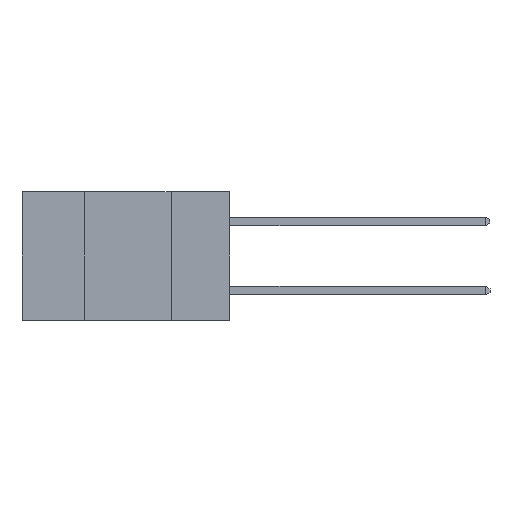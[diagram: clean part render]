
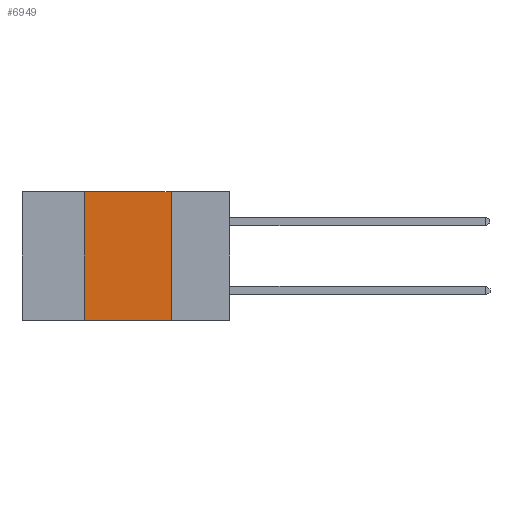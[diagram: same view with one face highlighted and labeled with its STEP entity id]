
A CAD part, left-side view. The second image highlights one B-rep face of the part: STEP entity #6949.
In plain terms, the highlighted planar face has unit normal (-1, 0, 0).
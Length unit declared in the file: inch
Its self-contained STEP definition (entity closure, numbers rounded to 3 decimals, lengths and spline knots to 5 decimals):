
#472 = VECTOR ( 'NONE', #587, 39.37008 ) ;
#587 = DIRECTION ( 'NONE',  ( 0., 0., -1. ) ) ;
#856 = CARTESIAN_POINT ( 'NONE',  ( 0., 0.6, 0. ) ) ;
#1259 = ORIENTED_EDGE ( 'NONE', *, *, #6615, .F. ) ;
#1535 = CARTESIAN_POINT ( 'NONE',  ( 0., 0.42, -0.37 ) ) ;
#1783 = VECTOR ( 'NONE', #5575, 39.37008 ) ;
#3051 = CARTESIAN_POINT ( 'NONE',  ( 0., 0.42, -0.37 ) ) ;
#3901 = DIRECTION ( 'NONE',  ( 0., -1., 0. ) ) ;
#3947 = LINE ( 'NONE', #3051, #8291 ) ;
#4255 = ORIENTED_EDGE ( 'NONE', *, *, #5945, .F. ) ;
#4301 = DIRECTION ( 'NONE',  ( 1., 0., 0. ) ) ;
#4339 = VERTEX_POINT ( 'NONE', #1535 ) ;
#4777 = LINE ( 'NONE', #9159, #472 ) ;
#5204 = EDGE_CURVE ( 'NONE', #4339, #5522, #6720, .T. ) ;
#5350 = EDGE_CURVE ( 'NONE', #5360, #5522, #4777, .T. ) ;
#5360 = VERTEX_POINT ( 'NONE', #7502 ) ;
#5522 = VERTEX_POINT ( 'NONE', #11032 ) ;
#5575 = DIRECTION ( 'NONE',  ( 0., -1., 0. ) ) ;
#5828 = ORIENTED_EDGE ( 'NONE', *, *, #5204, .T. ) ;
#5945 = EDGE_CURVE ( 'NONE', #4339, #7192, #3947, .T. ) ;
#6615 = EDGE_CURVE ( 'NONE', #7192, #5360, #10874, .T. ) ;
#6720 = LINE ( 'NONE', #9827, #1783 ) ;
#6949 = ADVANCED_FACE ( 'NONE', ( #9704 ), #9466, .F. ) ;
#7192 = VERTEX_POINT ( 'NONE', #8089 ) ;
#7502 = CARTESIAN_POINT ( 'NONE',  ( 0., 0.17, 0. ) ) ;
#7827 = ORIENTED_EDGE ( 'NONE', *, *, #5350, .F. ) ;
#8089 = CARTESIAN_POINT ( 'NONE',  ( 0., 0.42, 0. ) ) ;
#8291 = VECTOR ( 'NONE', #9081, 39.37008 ) ;
#9070 = CARTESIAN_POINT ( 'NONE',  ( 0., 0.6, 0. ) ) ;
#9081 = DIRECTION ( 'NONE',  ( 0., 0., 1. ) ) ;
#9159 = CARTESIAN_POINT ( 'NONE',  ( 0., 0.17, -0.37 ) ) ;
#9247 = AXIS2_PLACEMENT_3D ( 'NONE', #856, #4301, #10282 ) ;
#9466 = PLANE ( 'NONE',  #9247 ) ;
#9704 = FACE_OUTER_BOUND ( 'NONE', #10390, .T. ) ;
#9827 = CARTESIAN_POINT ( 'NONE',  ( 0., 0.6, -0.37 ) ) ;
#10282 = DIRECTION ( 'NONE',  ( 0., 0., -1. ) ) ;
#10390 = EDGE_LOOP ( 'NONE', ( #7827, #1259, #4255, #5828 ) ) ;
#10610 = VECTOR ( 'NONE', #3901, 39.37008 ) ;
#10874 = LINE ( 'NONE', #9070, #10610 ) ;
#11032 = CARTESIAN_POINT ( 'NONE',  ( 0., 0.17, -0.37 ) ) ;
